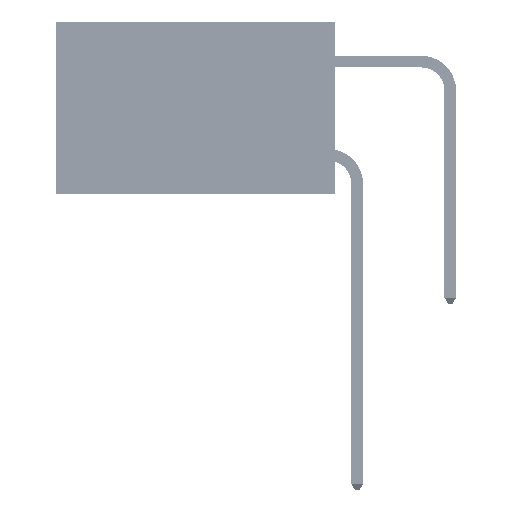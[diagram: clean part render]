
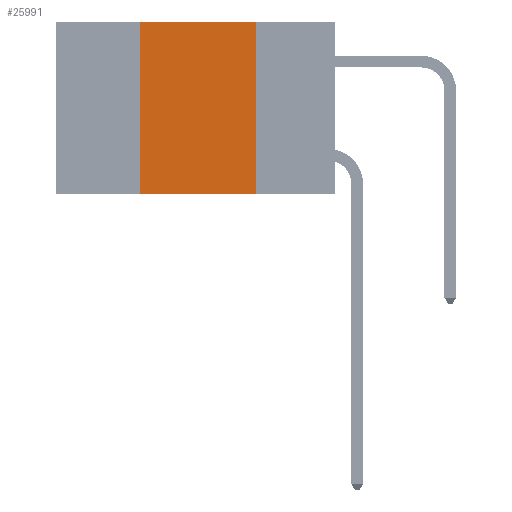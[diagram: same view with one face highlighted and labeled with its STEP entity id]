
A CAD part, left-side view. The second image highlights one B-rep face of the part: STEP entity #25991.
In plain terms, the highlighted planar face has unit normal (-1, 0, 0).
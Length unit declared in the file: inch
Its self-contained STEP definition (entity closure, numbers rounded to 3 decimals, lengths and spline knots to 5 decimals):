
#1928 = DIRECTION ( 'NONE',  ( 0., 0., -1. ) ) ;
#4831 = EDGE_CURVE ( 'NONE', #10108, #40747, #37678, .T. ) ;
#7479 = LINE ( 'NONE', #35468, #28257 ) ;
#7631 = LINE ( 'NONE', #38954, #50294 ) ;
#7945 = CARTESIAN_POINT ( 'NONE',  ( 0., 0.42, -0.37 ) ) ;
#9456 = CARTESIAN_POINT ( 'NONE',  ( 0., 0.6, 0. ) ) ;
#9946 = ORIENTED_EDGE ( 'NONE', *, *, #4831, .F. ) ;
#10108 = VERTEX_POINT ( 'NONE', #25174 ) ;
#12873 = LINE ( 'NONE', #35072, #32316 ) ;
#13650 = PLANE ( 'NONE',  #16259 ) ;
#14354 = VECTOR ( 'NONE', #25149, 39.37008 ) ;
#14869 = DIRECTION ( 'NONE',  ( 0., -1., 0. ) ) ;
#16259 = AXIS2_PLACEMENT_3D ( 'NONE', #9456, #17819, #46705 ) ;
#17819 = DIRECTION ( 'NONE',  ( 1., 0., 0. ) ) ;
#18507 = DIRECTION ( 'NONE',  ( 0., 0., 1. ) ) ;
#20306 = ORIENTED_EDGE ( 'NONE', *, *, #48935, .F. ) ;
#22952 = FACE_OUTER_BOUND ( 'NONE', #27458, .T. ) ;
#25149 = DIRECTION ( 'NONE',  ( 0., -1., 0. ) ) ;
#25174 = CARTESIAN_POINT ( 'NONE',  ( 0., 0.42, 0. ) ) ;
#25991 = ADVANCED_FACE ( 'NONE', ( #22952 ), #13650, .F. ) ;
#26761 = VERTEX_POINT ( 'NONE', #30777 ) ;
#26941 = ORIENTED_EDGE ( 'NONE', *, *, #50291, .T. ) ;
#27458 = EDGE_LOOP ( 'NONE', ( #20306, #9946, #32077, #26941 ) ) ;
#28257 = VECTOR ( 'NONE', #14869, 39.37008 ) ;
#30777 = CARTESIAN_POINT ( 'NONE',  ( 0., 0.17, -0.37 ) ) ;
#32077 = ORIENTED_EDGE ( 'NONE', *, *, #32395, .F. ) ;
#32316 = VECTOR ( 'NONE', #1928, 39.37008 ) ;
#32395 = EDGE_CURVE ( 'NONE', #36313, #10108, #7631, .T. ) ;
#35072 = CARTESIAN_POINT ( 'NONE',  ( 0., 0.17, 0. ) ) ;
#35468 = CARTESIAN_POINT ( 'NONE',  ( 0., 0.6, -0.37 ) ) ;
#36313 = VERTEX_POINT ( 'NONE', #7945 ) ;
#36323 = CARTESIAN_POINT ( 'NONE',  ( 0., 0.17, 0. ) ) ;
#37678 = LINE ( 'NONE', #41582, #14354 ) ;
#38954 = CARTESIAN_POINT ( 'NONE',  ( 0., 0.42, 0. ) ) ;
#40747 = VERTEX_POINT ( 'NONE', #36323 ) ;
#41582 = CARTESIAN_POINT ( 'NONE',  ( 0., 0.6, 0. ) ) ;
#46705 = DIRECTION ( 'NONE',  ( 0., 0., -1. ) ) ;
#48935 = EDGE_CURVE ( 'NONE', #40747, #26761, #12873, .T. ) ;
#50291 = EDGE_CURVE ( 'NONE', #36313, #26761, #7479, .T. ) ;
#50294 = VECTOR ( 'NONE', #18507, 39.37008 ) ;
